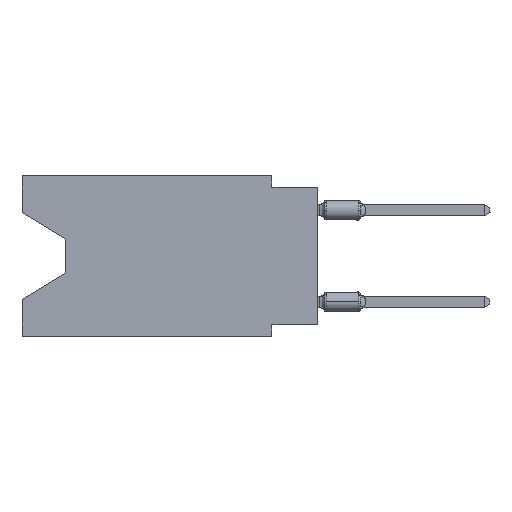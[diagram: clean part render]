
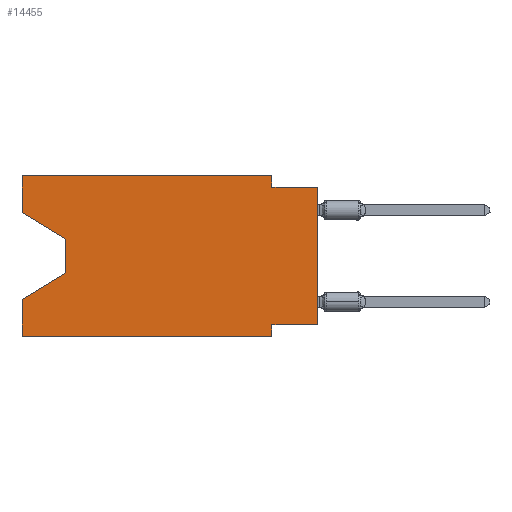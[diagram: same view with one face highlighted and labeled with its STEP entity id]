
A CAD part, left-side view. The second image highlights one B-rep face of the part: STEP entity #14455.
In plain terms, the highlighted planar face has unit normal (-1, 0, 0).
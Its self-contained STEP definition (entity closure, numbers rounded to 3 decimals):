
#225 = CARTESIAN_POINT ( 'NONE',  ( 0., 13.97, -3.505 ) ) ;
#559 = LINE ( 'NONE', #6729, #59436 ) ;
#1937 = VERTEX_POINT ( 'NONE', #33041 ) ;
#3219 = ORIENTED_EDGE ( 'NONE', *, *, #21528, .F. ) ;
#4585 = LINE ( 'NONE', #11157, #66570 ) ;
#4724 = VERTEX_POINT ( 'NONE', #19159 ) ;
#6053 = LINE ( 'NONE', #43954, #7333 ) ;
#6263 = VECTOR ( 'NONE', #62342, 1000. ) ;
#6729 = CARTESIAN_POINT ( 'NONE',  ( 0., 2.54, -8.89 ) ) ;
#7333 = VECTOR ( 'NONE', #49059, 1000. ) ;
#8217 = CARTESIAN_POINT ( 'NONE',  ( 0., 0., -0.635 ) ) ;
#8487 = VECTOR ( 'NONE', #42036, 1000. ) ;
#8740 = DIRECTION ( 'NONE',  ( 1., 0., 0. ) ) ;
#9602 = CARTESIAN_POINT ( 'NONE',  ( 0., 2.54, 0. ) ) ;
#9678 = ORIENTED_EDGE ( 'NONE', *, *, #55079, .T. ) ;
#10140 = EDGE_CURVE ( 'NONE', #34435, #65391, #31153, .T. ) ;
#10421 = LINE ( 'NONE', #225, #49518 ) ;
#10451 = VECTOR ( 'NONE', #65678, 1000. ) ;
#11157 = CARTESIAN_POINT ( 'NONE',  ( 0., 16.383, 0. ) ) ;
#11531 = VECTOR ( 'NONE', #13929, 1000. ) ;
#11689 = CARTESIAN_POINT ( 'NONE',  ( 0., 0., -8.255 ) ) ;
#12368 = ORIENTED_EDGE ( 'NONE', *, *, #71852, .T. ) ;
#13339 = EDGE_CURVE ( 'NONE', #50548, #45543, #31958, .T. ) ;
#13816 = CARTESIAN_POINT ( 'NONE',  ( 0., 16.383, -8.89 ) ) ;
#13929 = DIRECTION ( 'NONE',  ( 0., -0.855, -0.519 ) ) ;
#14455 = ADVANCED_FACE ( 'NONE', ( #51050 ), #47728, .F. ) ;
#14482 = CARTESIAN_POINT ( 'NONE',  ( 0., 16.383, 0. ) ) ;
#16760 = ORIENTED_EDGE ( 'NONE', *, *, #40542, .F. ) ;
#17244 = CARTESIAN_POINT ( 'NONE',  ( 0., 2.54, -0.635 ) ) ;
#17397 = ORIENTED_EDGE ( 'NONE', *, *, #51029, .F. ) ;
#19106 = LINE ( 'NONE', #69401, #8487 ) ;
#19159 = CARTESIAN_POINT ( 'NONE',  ( 0., 2.54, -8.255 ) ) ;
#19413 = LINE ( 'NONE', #31047, #11531 ) ;
#20370 = CARTESIAN_POINT ( 'NONE',  ( 0., 0., -8.255 ) ) ;
#21304 = ORIENTED_EDGE ( 'NONE', *, *, #67128, .F. ) ;
#21495 = VECTOR ( 'NONE', #24989, 1000. ) ;
#21528 = EDGE_CURVE ( 'NONE', #64205, #4724, #66399, .T. ) ;
#22521 = VERTEX_POINT ( 'NONE', #51129 ) ;
#24179 = EDGE_CURVE ( 'NONE', #38609, #45543, #32110, .T. ) ;
#24989 = DIRECTION ( 'NONE',  ( 0., -1., 0. ) ) ;
#25288 = VECTOR ( 'NONE', #49608, 1000. ) ;
#25477 = CARTESIAN_POINT ( 'NONE',  ( 0., 0., -0.635 ) ) ;
#27540 = DIRECTION ( 'NONE',  ( 0., 0., -1. ) ) ;
#28019 = CARTESIAN_POINT ( 'NONE',  ( 0., 16.383, -8.89 ) ) ;
#30266 = VECTOR ( 'NONE', #62563, 1000. ) ;
#31047 = CARTESIAN_POINT ( 'NONE',  ( 0., 16.383, -2.038 ) ) ;
#31153 = LINE ( 'NONE', #8217, #21495 ) ;
#31688 = DIRECTION ( 'NONE',  ( 0., 0., -1. ) ) ;
#31958 = LINE ( 'NONE', #14482, #34951 ) ;
#32110 = LINE ( 'NONE', #60926, #10451 ) ;
#32988 = EDGE_LOOP ( 'NONE', ( #12368, #9678, #51353, #41127, #46517, #43180, #3219, #37164, #37508, #21304, #17397, #16760 ) ) ;
#33041 = CARTESIAN_POINT ( 'NONE',  ( 0., 2.54, -8.89 ) ) ;
#33387 = DIRECTION ( 'NONE',  ( 0., -1., 0. ) ) ;
#34435 = VERTEX_POINT ( 'NONE', #17244 ) ;
#34951 = VECTOR ( 'NONE', #59689, 1000. ) ;
#35270 = VERTEX_POINT ( 'NONE', #46712 ) ;
#35342 = LINE ( 'NONE', #13816, #6263 ) ;
#37144 = EDGE_CURVE ( 'NONE', #50548, #1937, #35342, .T. ) ;
#37164 = ORIENTED_EDGE ( 'NONE', *, *, #59402, .T. ) ;
#37508 = ORIENTED_EDGE ( 'NONE', *, *, #10140, .F. ) ;
#38609 = VERTEX_POINT ( 'NONE', #71748 ) ;
#38875 = CARTESIAN_POINT ( 'NONE',  ( 0., 0., 0. ) ) ;
#40542 = EDGE_CURVE ( 'NONE', #22521, #71828, #19106, .T. ) ;
#41127 = ORIENTED_EDGE ( 'NONE', *, *, #13339, .F. ) ;
#42036 = DIRECTION ( 'NONE',  ( 0., 0., 1. ) ) ;
#43180 = ORIENTED_EDGE ( 'NONE', *, *, #47844, .F. ) ;
#43954 = CARTESIAN_POINT ( 'NONE',  ( 0., 2.54, 0. ) ) ;
#45543 = VERTEX_POINT ( 'NONE', #51698 ) ;
#46517 = ORIENTED_EDGE ( 'NONE', *, *, #37144, .T. ) ;
#46712 = CARTESIAN_POINT ( 'NONE',  ( 0., 13.97, -3.505 ) ) ;
#47728 = PLANE ( 'NONE',  #64230 ) ;
#47844 = EDGE_CURVE ( 'NONE', #4724, #1937, #559, .T. ) ;
#49059 = DIRECTION ( 'NONE',  ( 0., 0., -1. ) ) ;
#49518 = VECTOR ( 'NONE', #61480, 1000. ) ;
#49608 = DIRECTION ( 'NONE',  ( 0., 1., 0. ) ) ;
#50548 = VERTEX_POINT ( 'NONE', #28019 ) ;
#50886 = LINE ( 'NONE', #38875, #30266 ) ;
#51029 = EDGE_CURVE ( 'NONE', #71828, #66342, #4585, .T. ) ;
#51050 = FACE_OUTER_BOUND ( 'NONE', #32988, .T. ) ;
#51129 = CARTESIAN_POINT ( 'NONE',  ( 0., 16.383, -2.038 ) ) ;
#51353 = ORIENTED_EDGE ( 'NONE', *, *, #24179, .T. ) ;
#51698 = CARTESIAN_POINT ( 'NONE',  ( 0., 16.383, -6.852 ) ) ;
#53285 = CARTESIAN_POINT ( 'NONE',  ( 0., 16.383, 0. ) ) ;
#53931 = CARTESIAN_POINT ( 'NONE',  ( 0., 16.383, 0. ) ) ;
#55079 = EDGE_CURVE ( 'NONE', #35270, #38609, #10421, .T. ) ;
#59402 = EDGE_CURVE ( 'NONE', #64205, #65391, #50886, .T. ) ;
#59436 = VECTOR ( 'NONE', #27540, 1000. ) ;
#59689 = DIRECTION ( 'NONE',  ( 0., 0., 1. ) ) ;
#60926 = CARTESIAN_POINT ( 'NONE',  ( 0., 13.97, -5.385 ) ) ;
#61480 = DIRECTION ( 'NONE',  ( 0., 0., -1. ) ) ;
#62342 = DIRECTION ( 'NONE',  ( 0., -1., 0. ) ) ;
#62563 = DIRECTION ( 'NONE',  ( 0., 0., 1. ) ) ;
#64205 = VERTEX_POINT ( 'NONE', #20370 ) ;
#64230 = AXIS2_PLACEMENT_3D ( 'NONE', #53931, #8740, #31688 ) ;
#65391 = VERTEX_POINT ( 'NONE', #25477 ) ;
#65678 = DIRECTION ( 'NONE',  ( 0., 0.855, -0.519 ) ) ;
#66342 = VERTEX_POINT ( 'NONE', #9602 ) ;
#66399 = LINE ( 'NONE', #11689, #25288 ) ;
#66570 = VECTOR ( 'NONE', #33387, 1000. ) ;
#67128 = EDGE_CURVE ( 'NONE', #66342, #34435, #6053, .T. ) ;
#69401 = CARTESIAN_POINT ( 'NONE',  ( 0., 16.383, 0. ) ) ;
#71748 = CARTESIAN_POINT ( 'NONE',  ( 0., 13.97, -5.385 ) ) ;
#71828 = VERTEX_POINT ( 'NONE', #53285 ) ;
#71852 = EDGE_CURVE ( 'NONE', #22521, #35270, #19413, .T. ) ;
